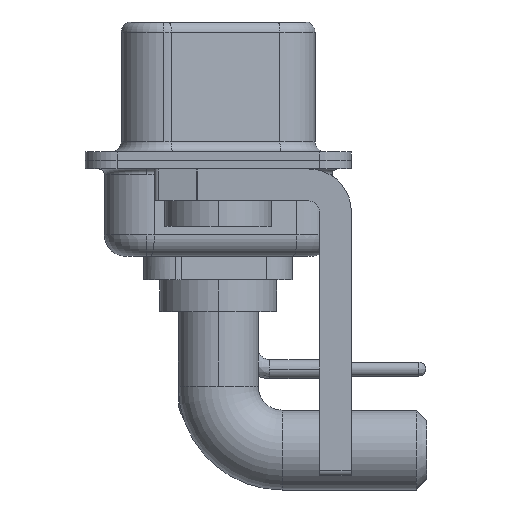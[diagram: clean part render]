
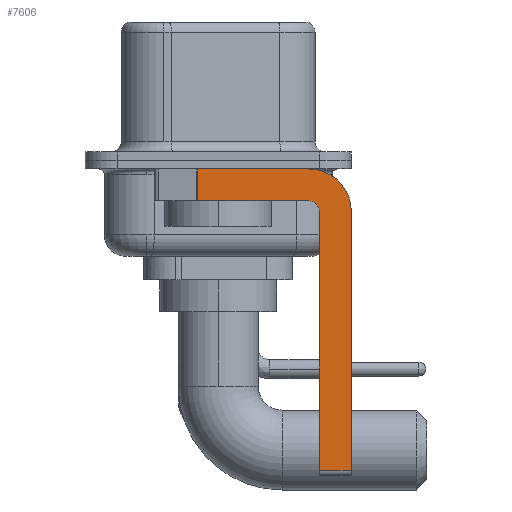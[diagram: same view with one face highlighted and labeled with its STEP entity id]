
A CAD part, left-side view. The second image highlights one B-rep face of the part: STEP entity #7606.
In plain terms, the highlighted planar face has unit normal (-1, 0, 0).
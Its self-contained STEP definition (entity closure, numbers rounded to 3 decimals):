
#277 = CIRCLE ( 'NONE', #15000, 0.5 ) ;
#997 = VECTOR ( 'NONE', #12122, 1000. ) ;
#1111 = VECTOR ( 'NONE', #16766, 1000. ) ;
#1424 = CARTESIAN_POINT ( 'NONE',  ( -2.9, 3., -0.4 ) ) ;
#2040 = DIRECTION ( 'NONE',  ( 0., 1., 0. ) ) ;
#3574 = ORIENTED_EDGE ( 'NONE', *, *, #17102, .F. ) ;
#3830 = DIRECTION ( 'NONE',  ( 1., 0., 0. ) ) ;
#4234 = VERTEX_POINT ( 'NONE', #18760 ) ;
#4341 = EDGE_CURVE ( 'NONE', #13146, #20616, #22884, .T. ) ;
#4616 = EDGE_CURVE ( 'NONE', #20616, #7616, #277, .T. ) ;
#5147 = DIRECTION ( 'NONE',  ( 0., 0., -1. ) ) ;
#5598 = PLANE ( 'NONE',  #14700 ) ;
#5652 = CARTESIAN_POINT ( 'NONE',  ( -2.9, -4.25, -0.4 ) ) ;
#5918 = CARTESIAN_POINT ( 'NONE',  ( -2.9, -4.25, -14.55 ) ) ;
#6347 = CARTESIAN_POINT ( 'NONE',  ( -2.9, -6.25, -2.4 ) ) ;
#6679 = CARTESIAN_POINT ( 'NONE',  ( -2.9, -4.75, -14.8 ) ) ;
#7019 = VERTEX_POINT ( 'NONE', #10483 ) ;
#7606 = ADVANCED_FACE ( 'NONE', ( #21815 ), #5598, .F. ) ;
#7616 = VERTEX_POINT ( 'NONE', #18717 ) ;
#7855 = EDGE_CURVE ( 'NONE', #17172, #11812, #15618, .T. ) ;
#7896 = LINE ( 'NONE', #6347, #1111 ) ;
#7929 = ORIENTED_EDGE ( 'NONE', *, *, #7855, .F. ) ;
#8165 = ORIENTED_EDGE ( 'NONE', *, *, #11979, .F. ) ;
#8221 = CARTESIAN_POINT ( 'NONE',  ( -2.9, 0.978, -1.9 ) ) ;
#8400 = CARTESIAN_POINT ( 'NONE',  ( -2.9, -4.75, -2.4 ) ) ;
#8959 = CARTESIAN_POINT ( 'NONE',  ( -2.9, -4.25, -2.4 ) ) ;
#9547 = CARTESIAN_POINT ( 'NONE',  ( -2.9, 0.978, -0.4 ) ) ;
#10451 = DIRECTION ( 'NONE',  ( 0., 0., -1. ) ) ;
#10483 = CARTESIAN_POINT ( 'NONE',  ( -2.9, -6.25, -14.55 ) ) ;
#11176 = DIRECTION ( 'NONE',  ( 0., 0., -1. ) ) ;
#11496 = VECTOR ( 'NONE', #13616, 1000. ) ;
#11609 = LINE ( 'NONE', #5918, #15212 ) ;
#11812 = VERTEX_POINT ( 'NONE', #5652 ) ;
#11979 = EDGE_CURVE ( 'NONE', #4234, #7019, #7896, .T. ) ;
#11985 = LINE ( 'NONE', #21196, #13593 ) ;
#12122 = DIRECTION ( 'NONE',  ( 0., 0., 1. ) ) ;
#12814 = CARTESIAN_POINT ( 'NONE',  ( -2.9, -4.25, -2.4 ) ) ;
#12874 = ORIENTED_EDGE ( 'NONE', *, *, #4616, .F. ) ;
#13146 = VERTEX_POINT ( 'NONE', #17676 ) ;
#13189 = VERTEX_POINT ( 'NONE', #8221 ) ;
#13267 = DIRECTION ( 'NONE',  ( 0., 0., 1. ) ) ;
#13334 = ORIENTED_EDGE ( 'NONE', *, *, #20153, .T. ) ;
#13593 = VECTOR ( 'NONE', #10451, 1000. ) ;
#13616 = DIRECTION ( 'NONE',  ( 0., -1., 0. ) ) ;
#14212 = CARTESIAN_POINT ( 'NONE',  ( -2.9, -4.25, -1.9 ) ) ;
#14700 = AXIS2_PLACEMENT_3D ( 'NONE', #12814, #3830, #11176 ) ;
#15000 = AXIS2_PLACEMENT_3D ( 'NONE', #22601, #17158, #13267 ) ;
#15212 = VECTOR ( 'NONE', #22361, 1000. ) ;
#15618 = LINE ( 'NONE', #1424, #11496 ) ;
#15900 = ORIENTED_EDGE ( 'NONE', *, *, #4341, .F. ) ;
#16134 = EDGE_CURVE ( 'NONE', #7616, #13189, #16209, .T. ) ;
#16209 = LINE ( 'NONE', #14212, #18596 ) ;
#16340 = EDGE_CURVE ( 'NONE', #13146, #7019, #11609, .T. ) ;
#16766 = DIRECTION ( 'NONE',  ( 0., 0., -1. ) ) ;
#17102 = EDGE_CURVE ( 'NONE', #11812, #4234, #20156, .T. ) ;
#17158 = DIRECTION ( 'NONE',  ( -1., 0., 0. ) ) ;
#17172 = VERTEX_POINT ( 'NONE', #9547 ) ;
#17584 = DIRECTION ( 'NONE',  ( 1., 0., 0. ) ) ;
#17676 = CARTESIAN_POINT ( 'NONE',  ( -2.9, -4.75, -14.55 ) ) ;
#18207 = ORIENTED_EDGE ( 'NONE', *, *, #16134, .F. ) ;
#18596 = VECTOR ( 'NONE', #2040, 1000. ) ;
#18717 = CARTESIAN_POINT ( 'NONE',  ( -2.9, -4.25, -1.9 ) ) ;
#18760 = CARTESIAN_POINT ( 'NONE',  ( -2.9, -6.25, -2.4 ) ) ;
#20144 = EDGE_LOOP ( 'NONE', ( #7929, #13334, #18207, #12874, #15900, #21930, #8165, #3574 ) ) ;
#20153 = EDGE_CURVE ( 'NONE', #17172, #13189, #11985, .T. ) ;
#20156 = CIRCLE ( 'NONE', #20891, 2. ) ;
#20616 = VERTEX_POINT ( 'NONE', #8400 ) ;
#20891 = AXIS2_PLACEMENT_3D ( 'NONE', #8959, #17584, #5147 ) ;
#21196 = CARTESIAN_POINT ( 'NONE',  ( -2.9, 0.978, -1.9 ) ) ;
#21815 = FACE_OUTER_BOUND ( 'NONE', #20144, .T. ) ;
#21930 = ORIENTED_EDGE ( 'NONE', *, *, #16340, .T. ) ;
#22361 = DIRECTION ( 'NONE',  ( 0., -1., 0. ) ) ;
#22601 = CARTESIAN_POINT ( 'NONE',  ( -2.9, -4.25, -2.4 ) ) ;
#22884 = LINE ( 'NONE', #6679, #997 ) ;
